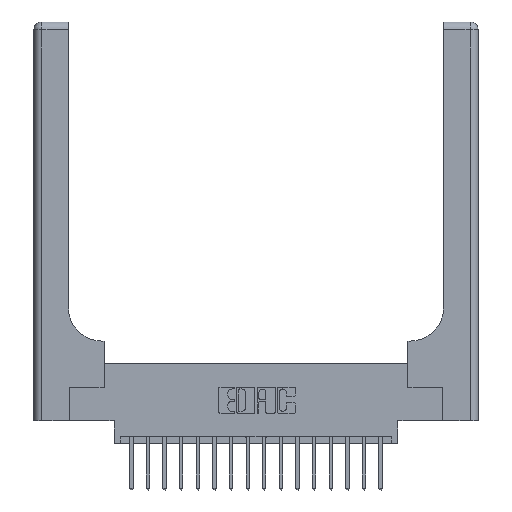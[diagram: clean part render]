
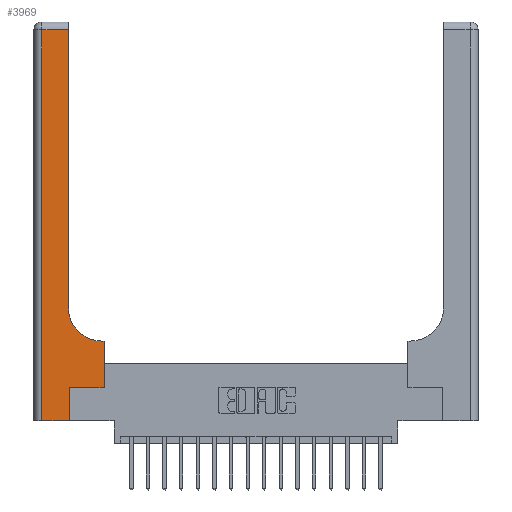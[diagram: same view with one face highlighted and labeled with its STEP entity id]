
A CAD part, top view. The second image highlights one B-rep face of the part: STEP entity #3969.
In plain terms, the highlighted planar face has unit normal (0, 0, 1).
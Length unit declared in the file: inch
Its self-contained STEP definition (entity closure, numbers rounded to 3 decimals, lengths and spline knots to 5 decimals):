
#132 = CARTESIAN_POINT ( 'NONE',  ( 0.528, 0.25, 0.37 ) ) ;
#296 = CARTESIAN_POINT ( 'NONE',  ( 0.26, 2.94, 0.37 ) ) ;
#333 = EDGE_CURVE ( 'NONE', #6853, #16306, #16228, .T. ) ;
#388 = VECTOR ( 'NONE', #2474, 39.37008 ) ;
#426 = CARTESIAN_POINT ( 'NONE',  ( 0.06, 3., 0.37 ) ) ;
#801 = CARTESIAN_POINT ( 'NONE',  ( 0.51, 0.6, 0.37 ) ) ;
#867 = ORIENTED_EDGE ( 'NONE', *, *, #1067, .T. ) ;
#1067 = EDGE_CURVE ( 'NONE', #1289, #10696, #13683, .T. ) ;
#1289 = VERTEX_POINT ( 'NONE', #13634 ) ;
#1471 = ORIENTED_EDGE ( 'NONE', *, *, #4193, .T. ) ;
#2474 = DIRECTION ( 'NONE',  ( -1., 0., 0. ) ) ;
#3368 = PLANE ( 'NONE',  #16957 ) ;
#3954 = VECTOR ( 'NONE', #8393, 39.37008 ) ;
#3969 = ADVANCED_FACE ( 'NONE', ( #4285 ), #3368, .F. ) ;
#4188 = VERTEX_POINT ( 'NONE', #6806 ) ;
#4193 = EDGE_CURVE ( 'NONE', #10426, #6853, #4508, .T. ) ;
#4285 = FACE_OUTER_BOUND ( 'NONE', #13492, .T. ) ;
#4313 = ORIENTED_EDGE ( 'NONE', *, *, #10460, .T. ) ;
#4508 = LINE ( 'NONE', #9813, #7995 ) ;
#4568 = LINE ( 'NONE', #426, #19031 ) ;
#4611 = VECTOR ( 'NONE', #18068, 39.37008 ) ;
#4873 = CARTESIAN_POINT ( 'NONE',  ( 0., 3., 0.37 ) ) ;
#5222 = DIRECTION ( 'NONE',  ( 0., 0., -1. ) ) ;
#5352 = LINE ( 'NONE', #15818, #3954 ) ;
#5881 = DIRECTION ( 'NONE',  ( -1., 0., 0. ) ) ;
#5952 = ORIENTED_EDGE ( 'NONE', *, *, #8226, .T. ) ;
#6180 = VECTOR ( 'NONE', #10536, 39.37008 ) ;
#6349 = DIRECTION ( 'NONE',  ( 0., 0., -1. ) ) ;
#6595 = EDGE_CURVE ( 'NONE', #17112, #11194, #5352, .T. ) ;
#6791 = LINE ( 'NONE', #9762, #10295 ) ;
#6806 = CARTESIAN_POINT ( 'NONE',  ( 0.528, 0.25, 0.37 ) ) ;
#6853 = VERTEX_POINT ( 'NONE', #296 ) ;
#6860 = VERTEX_POINT ( 'NONE', #7774 ) ;
#7095 = ORIENTED_EDGE ( 'NONE', *, *, #18329, .T. ) ;
#7774 = CARTESIAN_POINT ( 'NONE',  ( 0.265, 0.25, 0.37 ) ) ;
#7995 = VECTOR ( 'NONE', #11296, 39.37008 ) ;
#8058 = ORIENTED_EDGE ( 'NONE', *, *, #333, .T. ) ;
#8226 = EDGE_CURVE ( 'NONE', #6860, #4188, #6791, .T. ) ;
#8375 = ORIENTED_EDGE ( 'NONE', *, *, #19198, .T. ) ;
#8393 = DIRECTION ( 'NONE',  ( 1., 0., 0. ) ) ;
#9700 = CARTESIAN_POINT ( 'NONE',  ( 0.06, 0., 0.37 ) ) ;
#9715 = VECTOR ( 'NONE', #5881, 39.37008 ) ;
#9762 = CARTESIAN_POINT ( 'NONE',  ( 0.265, 0.25, 0.37 ) ) ;
#9766 = CARTESIAN_POINT ( 'NONE',  ( 0.265, 0., 0.37 ) ) ;
#9792 = ORIENTED_EDGE ( 'NONE', *, *, #10682, .T. ) ;
#9813 = CARTESIAN_POINT ( 'NONE',  ( 0.26, 3., 0.37 ) ) ;
#10295 = VECTOR ( 'NONE', #11248, 39.37008 ) ;
#10426 = VERTEX_POINT ( 'NONE', #12051 ) ;
#10460 = EDGE_CURVE ( 'NONE', #11194, #6860, #16487, .T. ) ;
#10528 = CARTESIAN_POINT ( 'NONE',  ( 0.06, 2.94, 0.37 ) ) ;
#10536 = DIRECTION ( 'NONE',  ( 0., 1., 0. ) ) ;
#10682 = EDGE_CURVE ( 'NONE', #10696, #10426, #16704, .T. ) ;
#10696 = VERTEX_POINT ( 'NONE', #801 ) ;
#11194 = VERTEX_POINT ( 'NONE', #9766 ) ;
#11248 = DIRECTION ( 'NONE',  ( 1., 0., 0. ) ) ;
#11296 = DIRECTION ( 'NONE',  ( 0., 1., 0. ) ) ;
#11384 = CARTESIAN_POINT ( 'NONE',  ( 0., 2.94, 0.37 ) ) ;
#11811 = CARTESIAN_POINT ( 'NONE',  ( 0.26, 0.6, 0.37 ) ) ;
#12051 = CARTESIAN_POINT ( 'NONE',  ( 0.26, 0.85, 0.37 ) ) ;
#13492 = EDGE_LOOP ( 'NONE', ( #1471, #8058, #7095, #18314, #4313, #5952, #8375, #867, #9792 ) ) ;
#13634 = CARTESIAN_POINT ( 'NONE',  ( 0.528, 0.6, 0.37 ) ) ;
#13683 = LINE ( 'NONE', #11811, #9715 ) ;
#13905 = AXIS2_PLACEMENT_3D ( 'NONE', #14147, #5222, #15640 ) ;
#14147 = CARTESIAN_POINT ( 'NONE',  ( 0.51, 0.85, 0.37 ) ) ;
#15640 = DIRECTION ( 'NONE',  ( 1., 0., 0. ) ) ;
#15818 = CARTESIAN_POINT ( 'NONE',  ( 0., 0., 0.37 ) ) ;
#16228 = LINE ( 'NONE', #11384, #388 ) ;
#16306 = VERTEX_POINT ( 'NONE', #10528 ) ;
#16487 = LINE ( 'NONE', #16546, #4611 ) ;
#16546 = CARTESIAN_POINT ( 'NONE',  ( 0.265, 0., 0.37 ) ) ;
#16704 = CIRCLE ( 'NONE', #13905, 0.25 ) ;
#16770 = DIRECTION ( 'NONE',  ( -1., 0., 0. ) ) ;
#16957 = AXIS2_PLACEMENT_3D ( 'NONE', #4873, #6349, #16770 ) ;
#17112 = VERTEX_POINT ( 'NONE', #9700 ) ;
#17132 = LINE ( 'NONE', #132, #6180 ) ;
#18068 = DIRECTION ( 'NONE',  ( 0., 1., 0. ) ) ;
#18269 = DIRECTION ( 'NONE',  ( 0., -1., 0. ) ) ;
#18314 = ORIENTED_EDGE ( 'NONE', *, *, #6595, .T. ) ;
#18329 = EDGE_CURVE ( 'NONE', #16306, #17112, #4568, .T. ) ;
#19031 = VECTOR ( 'NONE', #18269, 39.37008 ) ;
#19198 = EDGE_CURVE ( 'NONE', #4188, #1289, #17132, .T. ) ;
